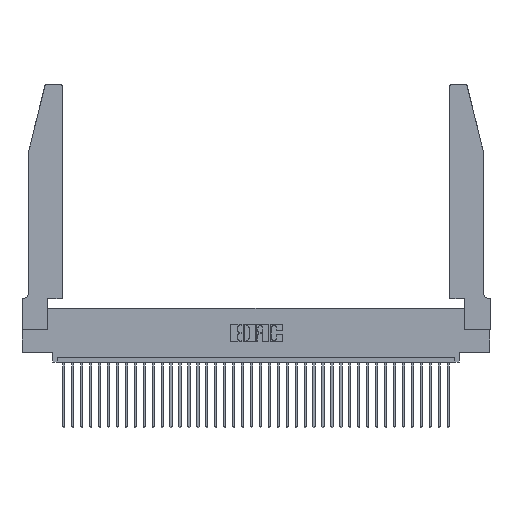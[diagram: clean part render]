
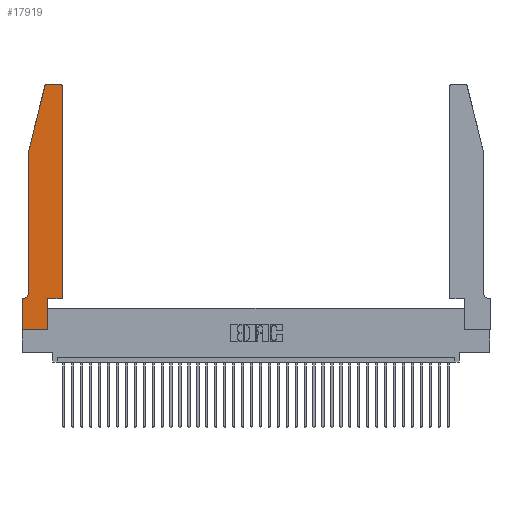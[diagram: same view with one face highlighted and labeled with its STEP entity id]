
A CAD part, top view. The second image highlights one B-rep face of the part: STEP entity #17919.
In plain terms, the highlighted planar face has unit normal (0, 0, 1).
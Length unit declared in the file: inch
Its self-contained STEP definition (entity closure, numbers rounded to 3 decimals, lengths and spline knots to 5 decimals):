
#4 = EDGE_CURVE ( 'NONE', #34717, #412, #33654, .T. ) ;
#412 = VERTEX_POINT ( 'NONE', #3652 ) ;
#696 = CARTESIAN_POINT ( 'NONE',  ( 0.4505, 2.72, 0.37 ) ) ;
#718 = DIRECTION ( 'NONE',  ( 0., 0., 1. ) ) ;
#3139 = CARTESIAN_POINT ( 'NONE',  ( 0.0755, 2., 0.37 ) ) ;
#3527 = CARTESIAN_POINT ( 'NONE',  ( 0.284, 2.72, 0.37 ) ) ;
#3652 = CARTESIAN_POINT ( 'NONE',  ( 0.4505, 0.35, 0.37 ) ) ;
#3666 = DIRECTION ( 'NONE',  ( 1., 0., 0. ) ) ;
#3949 = CIRCLE ( 'NONE', #15614, 0.03 ) ;
#4603 = CARTESIAN_POINT ( 'NONE',  ( 0.25487, 2.72718, 0.37 ) ) ;
#4819 = CARTESIAN_POINT ( 'NONE',  ( 0., 0.35, 0.37 ) ) ;
#5592 = DIRECTION ( 'NONE',  ( 0., 0., 1. ) ) ;
#5614 = VERTEX_POINT ( 'NONE', #4819 ) ;
#6228 = CARTESIAN_POINT ( 'NONE',  ( 0., 0., 0.37 ) ) ;
#7560 = CARTESIAN_POINT ( 'NONE',  ( 0.2865, 0.35, 0.37 ) ) ;
#7585 = EDGE_LOOP ( 'NONE', ( #10306, #31566, #7794, #31534, #23612, #15412, #13349, #29841, #17476, #14290, #19074, #17138 ) ) ;
#7794 = ORIENTED_EDGE ( 'NONE', *, *, #21647, .T. ) ;
#8219 = DIRECTION ( 'NONE',  ( -1., 0., 0. ) ) ;
#8612 = VERTEX_POINT ( 'NONE', #696 ) ;
#8721 = DIRECTION ( 'NONE',  ( 0., 1., 0. ) ) ;
#9053 = VERTEX_POINT ( 'NONE', #26854 ) ;
#9107 = CARTESIAN_POINT ( 'NONE',  ( 0.2605, 2.75, 0.37 ) ) ;
#9117 = DIRECTION ( 'NONE',  ( 0., -1., 0. ) ) ;
#10109 = VECTOR ( 'NONE', #8721, 39.37008 ) ;
#10116 = LINE ( 'NONE', #3139, #27970 ) ;
#10306 = ORIENTED_EDGE ( 'NONE', *, *, #22834, .T. ) ;
#10318 = PLANE ( 'NONE',  #17613 ) ;
#11548 = CARTESIAN_POINT ( 'NONE',  ( 0., 0., 0.37 ) ) ;
#13349 = ORIENTED_EDGE ( 'NONE', *, *, #19662, .T. ) ;
#13616 = CARTESIAN_POINT ( 'NONE',  ( 0.4505, 0.35, 0.37 ) ) ;
#14290 = ORIENTED_EDGE ( 'NONE', *, *, #4, .T. ) ;
#14329 = VECTOR ( 'NONE', #35040, 39.37008 ) ;
#14388 = EDGE_CURVE ( 'NONE', #25929, #5614, #27591, .T. ) ;
#14392 = DIRECTION ( 'NONE',  ( 0., 0., -1. ) ) ;
#14431 = VECTOR ( 'NONE', #34032, 39.37008 ) ;
#15412 = ORIENTED_EDGE ( 'NONE', *, *, #14388, .T. ) ;
#15568 = AXIS2_PLACEMENT_3D ( 'NONE', #37224, #14392, #8219 ) ;
#15614 = AXIS2_PLACEMENT_3D ( 'NONE', #37417, #5592, #19976 ) ;
#15617 = DIRECTION ( 'NONE',  ( 0., -1., 0. ) ) ;
#15972 = CARTESIAN_POINT ( 'NONE',  ( 0.2865, 0., 0.37 ) ) ;
#16602 = DIRECTION ( 'NONE',  ( 0., 1., 0. ) ) ;
#16661 = DIRECTION ( 'NONE',  ( 0., 0., 1. ) ) ;
#16916 = EDGE_CURVE ( 'NONE', #9053, #27644, #10116, .T. ) ;
#17138 = ORIENTED_EDGE ( 'NONE', *, *, #31681, .T. ) ;
#17476 = ORIENTED_EDGE ( 'NONE', *, *, #18435, .T. ) ;
#17613 = AXIS2_PLACEMENT_3D ( 'NONE', #30734, #16661, #35414 ) ;
#17919 = ADVANCED_FACE ( 'NONE', ( #27396 ), #10318, .T. ) ;
#18435 = EDGE_CURVE ( 'NONE', #22970, #34717, #35077, .T. ) ;
#18874 = CARTESIAN_POINT ( 'NONE',  ( 0.4205, 2.75, 0.37 ) ) ;
#19037 = CIRCLE ( 'NONE', #22081, 0.03 ) ;
#19074 = ORIENTED_EDGE ( 'NONE', *, *, #27646, .T. ) ;
#19662 = EDGE_CURVE ( 'NONE', #5614, #34050, #35912, .T. ) ;
#19936 = LINE ( 'NONE', #6228, #21773 ) ;
#19976 = DIRECTION ( 'NONE',  ( 1., 0., 0. ) ) ;
#20080 = EDGE_CURVE ( 'NONE', #27644, #25929, #37736, .T. ) ;
#20329 = CARTESIAN_POINT ( 'NONE',  ( 0., 0., 0.37 ) ) ;
#20571 = VERTEX_POINT ( 'NONE', #36148 ) ;
#21221 = VERTEX_POINT ( 'NONE', #18874 ) ;
#21647 = EDGE_CURVE ( 'NONE', #31462, #9053, #35101, .T. ) ;
#21773 = VECTOR ( 'NONE', #3666, 39.37008 ) ;
#22081 = AXIS2_PLACEMENT_3D ( 'NONE', #3527, #718, #23930 ) ;
#22458 = CARTESIAN_POINT ( 'NONE',  ( 0.0755, 0.35, 0.37 ) ) ;
#22741 = CARTESIAN_POINT ( 'NONE',  ( 0.4505, 0.35, 0.37 ) ) ;
#22834 = EDGE_CURVE ( 'NONE', #21221, #20571, #27337, .T. ) ;
#22970 = VERTEX_POINT ( 'NONE', #15972 ) ;
#23237 = VECTOR ( 'NONE', #30496, 39.37008 ) ;
#23612 = ORIENTED_EDGE ( 'NONE', *, *, #20080, .T. ) ;
#23661 = VECTOR ( 'NONE', #29498, 39.37008 ) ;
#23930 = DIRECTION ( 'NONE',  ( 1., 0., 0. ) ) ;
#24072 = EDGE_CURVE ( 'NONE', #20571, #31462, #19037, .T. ) ;
#25446 = VECTOR ( 'NONE', #9117, 39.37008 ) ;
#25929 = VERTEX_POINT ( 'NONE', #26435 ) ;
#26435 = CARTESIAN_POINT ( 'NONE',  ( 0.0055, 0.35, 0.37 ) ) ;
#26854 = CARTESIAN_POINT ( 'NONE',  ( 0.0755, 2., 0.37 ) ) ;
#27337 = LINE ( 'NONE', #9107, #23661 ) ;
#27396 = FACE_OUTER_BOUND ( 'NONE', #7585, .T. ) ;
#27457 = LINE ( 'NONE', #22741, #10109 ) ;
#27591 = LINE ( 'NONE', #22458, #14329 ) ;
#27644 = VERTEX_POINT ( 'NONE', #29228 ) ;
#27646 = EDGE_CURVE ( 'NONE', #412, #8612, #27457, .T. ) ;
#27970 = VECTOR ( 'NONE', #15617, 39.37008 ) ;
#29228 = CARTESIAN_POINT ( 'NONE',  ( 0.0755, 0.42, 0.37 ) ) ;
#29498 = DIRECTION ( 'NONE',  ( -1., 0., 0. ) ) ;
#29841 = ORIENTED_EDGE ( 'NONE', *, *, #31184, .T. ) ;
#29981 = CARTESIAN_POINT ( 'NONE',  ( 0.0755, 2., 0.37 ) ) ;
#30496 = DIRECTION ( 'NONE',  ( -0.239, -0.971, 0. ) ) ;
#30734 = CARTESIAN_POINT ( 'NONE',  ( 0., 0.35, 0.37 ) ) ;
#31184 = EDGE_CURVE ( 'NONE', #34050, #22970, #19936, .T. ) ;
#31462 = VERTEX_POINT ( 'NONE', #4603 ) ;
#31534 = ORIENTED_EDGE ( 'NONE', *, *, #16916, .T. ) ;
#31566 = ORIENTED_EDGE ( 'NONE', *, *, #24072, .T. ) ;
#31681 = EDGE_CURVE ( 'NONE', #8612, #21221, #3949, .T. ) ;
#33654 = LINE ( 'NONE', #13616, #14431 ) ;
#33749 = VECTOR ( 'NONE', #16602, 39.37008 ) ;
#34032 = DIRECTION ( 'NONE',  ( 1., 0., 0. ) ) ;
#34050 = VERTEX_POINT ( 'NONE', #20329 ) ;
#34717 = VERTEX_POINT ( 'NONE', #37371 ) ;
#35040 = DIRECTION ( 'NONE',  ( -1., 0., 0. ) ) ;
#35077 = LINE ( 'NONE', #7560, #33749 ) ;
#35101 = LINE ( 'NONE', #29981, #23237 ) ;
#35414 = DIRECTION ( 'NONE',  ( 1., 0., 0. ) ) ;
#35912 = LINE ( 'NONE', #11548, #25446 ) ;
#36148 = CARTESIAN_POINT ( 'NONE',  ( 0.284, 2.75, 0.37 ) ) ;
#37224 = CARTESIAN_POINT ( 'NONE',  ( 0.0055, 0.42, 0.37 ) ) ;
#37371 = CARTESIAN_POINT ( 'NONE',  ( 0.2865, 0.35, 0.37 ) ) ;
#37417 = CARTESIAN_POINT ( 'NONE',  ( 0.4205, 2.72, 0.37 ) ) ;
#37736 = CIRCLE ( 'NONE', #15568, 0.07 ) ;
